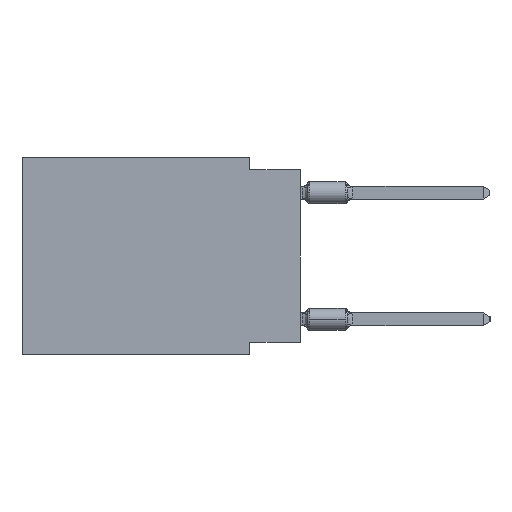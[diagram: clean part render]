
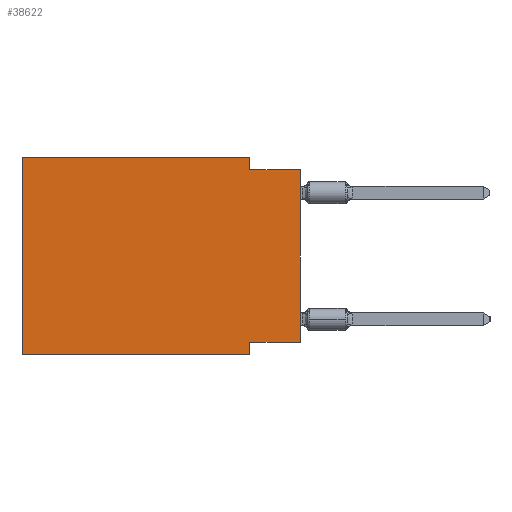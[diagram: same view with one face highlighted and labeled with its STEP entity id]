
A CAD part, left-side view. The second image highlights one B-rep face of the part: STEP entity #38622.
In plain terms, the highlighted planar face has unit normal (-1, 0, 0).
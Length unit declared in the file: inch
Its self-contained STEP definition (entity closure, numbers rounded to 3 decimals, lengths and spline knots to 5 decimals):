
#865 = VECTOR ( 'NONE', #16555, 39.37008 ) ;
#908 = EDGE_CURVE ( 'NONE', #36863, #15926, #28945, .T. ) ;
#1138 = VERTEX_POINT ( 'NONE', #20341 ) ;
#1188 = VECTOR ( 'NONE', #25306, 39.37008 ) ;
#1430 = CARTESIAN_POINT ( 'NONE',  ( 0., 0.55, 0. ) ) ;
#1758 = CARTESIAN_POINT ( 'NONE',  ( 0., 0.1, 0. ) ) ;
#5172 = EDGE_CURVE ( 'NONE', #8296, #19469, #13405, .T. ) ;
#5745 = VECTOR ( 'NONE', #45396, 39.37008 ) ;
#6158 = FACE_OUTER_BOUND ( 'NONE', #33140, .T. ) ;
#6513 = ORIENTED_EDGE ( 'NONE', *, *, #908, .T. ) ;
#6891 = ORIENTED_EDGE ( 'NONE', *, *, #36480, .F. ) ;
#8296 = VERTEX_POINT ( 'NONE', #24783 ) ;
#9074 = DIRECTION ( 'NONE',  ( 1., 0., 0. ) ) ;
#10042 = PLANE ( 'NONE',  #19874 ) ;
#13081 = EDGE_CURVE ( 'NONE', #1138, #16387, #16331, .T. ) ;
#13405 = LINE ( 'NONE', #1758, #865 ) ;
#13684 = CARTESIAN_POINT ( 'NONE',  ( 0., 0.55, 0. ) ) ;
#15167 = EDGE_CURVE ( 'NONE', #19469, #15926, #15757, .T. ) ;
#15669 = LINE ( 'NONE', #30494, #35346 ) ;
#15757 = LINE ( 'NONE', #16466, #5745 ) ;
#15926 = VERTEX_POINT ( 'NONE', #27985 ) ;
#16331 = LINE ( 'NONE', #38697, #42848 ) ;
#16387 = VERTEX_POINT ( 'NONE', #23205 ) ;
#16466 = CARTESIAN_POINT ( 'NONE',  ( 0., 0., -0.025 ) ) ;
#16555 = DIRECTION ( 'NONE',  ( 0., 0., -1. ) ) ;
#17969 = EDGE_CURVE ( 'NONE', #42390, #16387, #34786, .T. ) ;
#18340 = VECTOR ( 'NONE', #34081, 39.37008 ) ;
#19265 = CARTESIAN_POINT ( 'NONE',  ( 0., 0.1, -0.39 ) ) ;
#19418 = DIRECTION ( 'NONE',  ( 0., -1., 0. ) ) ;
#19469 = VERTEX_POINT ( 'NONE', #29512 ) ;
#19874 = AXIS2_PLACEMENT_3D ( 'NONE', #13684, #9074, #35561 ) ;
#20092 = CARTESIAN_POINT ( 'NONE',  ( 0., 0.55, 0. ) ) ;
#20341 = CARTESIAN_POINT ( 'NONE',  ( 0., 0.55, -0.39 ) ) ;
#21276 = ORIENTED_EDGE ( 'NONE', *, *, #27846, .F. ) ;
#23072 = LINE ( 'NONE', #1430, #44979 ) ;
#23205 = CARTESIAN_POINT ( 'NONE',  ( 0., 0.1, -0.39 ) ) ;
#23693 = VECTOR ( 'NONE', #43030, 39.37008 ) ;
#24783 = CARTESIAN_POINT ( 'NONE',  ( 0., 0.1, 0. ) ) ;
#25306 = DIRECTION ( 'NONE',  ( 0., 1., 0. ) ) ;
#26501 = ORIENTED_EDGE ( 'NONE', *, *, #5172, .F. ) ;
#27352 = ORIENTED_EDGE ( 'NONE', *, *, #17969, .F. ) ;
#27610 = CARTESIAN_POINT ( 'NONE',  ( 0., 0.1, -0.365 ) ) ;
#27846 = EDGE_CURVE ( 'NONE', #1138, #44938, #15669, .T. ) ;
#27985 = CARTESIAN_POINT ( 'NONE',  ( 0., 0., -0.025 ) ) ;
#28423 = ORIENTED_EDGE ( 'NONE', *, *, #15167, .F. ) ;
#28945 = LINE ( 'NONE', #43763, #23693 ) ;
#29512 = CARTESIAN_POINT ( 'NONE',  ( 0., 0.1, -0.025 ) ) ;
#29640 = EDGE_CURVE ( 'NONE', #36863, #42390, #43773, .T. ) ;
#30494 = CARTESIAN_POINT ( 'NONE',  ( 0., 0.55, 0. ) ) ;
#30922 = DIRECTION ( 'NONE',  ( 0., -1., 0. ) ) ;
#33140 = EDGE_LOOP ( 'NONE', ( #6513, #28423, #26501, #6891, #21276, #46893, #27352, #33280 ) ) ;
#33280 = ORIENTED_EDGE ( 'NONE', *, *, #29640, .F. ) ;
#34081 = DIRECTION ( 'NONE',  ( 0., 0., -1. ) ) ;
#34786 = LINE ( 'NONE', #19265, #18340 ) ;
#35346 = VECTOR ( 'NONE', #45310, 39.37008 ) ;
#35561 = DIRECTION ( 'NONE',  ( 0., 0., -1. ) ) ;
#36091 = CARTESIAN_POINT ( 'NONE',  ( 0., 0., -0.365 ) ) ;
#36480 = EDGE_CURVE ( 'NONE', #44938, #8296, #23072, .T. ) ;
#36489 = CARTESIAN_POINT ( 'NONE',  ( 0., 0., -0.365 ) ) ;
#36863 = VERTEX_POINT ( 'NONE', #36091 ) ;
#38622 = ADVANCED_FACE ( 'NONE', ( #6158 ), #10042, .F. ) ;
#38697 = CARTESIAN_POINT ( 'NONE',  ( 0., 0.55, -0.39 ) ) ;
#42390 = VERTEX_POINT ( 'NONE', #27610 ) ;
#42848 = VECTOR ( 'NONE', #30922, 39.37008 ) ;
#43030 = DIRECTION ( 'NONE',  ( 0., 0., 1. ) ) ;
#43763 = CARTESIAN_POINT ( 'NONE',  ( 0., 0., 0. ) ) ;
#43773 = LINE ( 'NONE', #36489, #1188 ) ;
#44938 = VERTEX_POINT ( 'NONE', #20092 ) ;
#44979 = VECTOR ( 'NONE', #19418, 39.37008 ) ;
#45310 = DIRECTION ( 'NONE',  ( 0., 0., 1. ) ) ;
#45396 = DIRECTION ( 'NONE',  ( 0., -1., 0. ) ) ;
#46893 = ORIENTED_EDGE ( 'NONE', *, *, #13081, .T. ) ;
